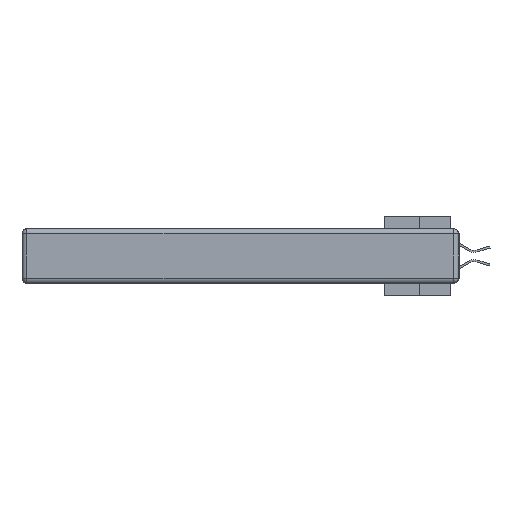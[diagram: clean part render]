
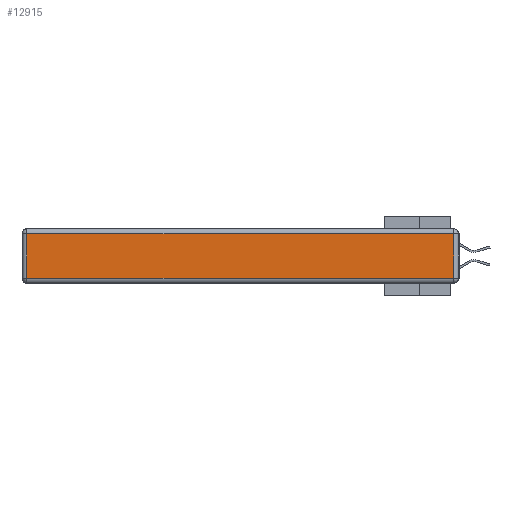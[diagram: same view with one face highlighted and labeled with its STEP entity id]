
A CAD part, left-side view. The second image highlights one B-rep face of the part: STEP entity #12915.
In plain terms, the highlighted planar face has unit normal (-1, 0, 0).
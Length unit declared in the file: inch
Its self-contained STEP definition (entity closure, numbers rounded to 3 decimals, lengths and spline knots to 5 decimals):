
#353 = EDGE_LOOP ( 'NONE', ( #5043, #460, #6641, #28069 ) ) ;
#437 = DIRECTION ( 'NONE',  ( -1., 0., 0. ) ) ;
#460 = ORIENTED_EDGE ( 'NONE', *, *, #6796, .T. ) ;
#1676 = FACE_OUTER_BOUND ( 'NONE', #353, .T. ) ;
#2303 = LINE ( 'NONE', #7377, #29376 ) ;
#2669 = PLANE ( 'NONE',  #26772 ) ;
#3069 = CARTESIAN_POINT ( 'NONE',  ( 0., 0., -0.343 ) ) ;
#3465 = VERTEX_POINT ( 'NONE', #5229 ) ;
#3587 = VECTOR ( 'NONE', #23182, 39.37008 ) ;
#4203 = CARTESIAN_POINT ( 'NONE',  ( 0., 0., -0.313 ) ) ;
#4297 = DIRECTION ( 'NONE',  ( 0., -1., 0. ) ) ;
#4678 = DIRECTION ( 'NONE',  ( 0., 1., 0. ) ) ;
#5043 = ORIENTED_EDGE ( 'NONE', *, *, #13978, .T. ) ;
#5229 = CARTESIAN_POINT ( 'NONE',  ( 0., 0.03, -0.313 ) ) ;
#5872 = VERTEX_POINT ( 'NONE', #11724 ) ;
#6641 = ORIENTED_EDGE ( 'NONE', *, *, #22964, .T. ) ;
#6796 = EDGE_CURVE ( 'NONE', #3465, #5872, #2303, .T. ) ;
#7377 = CARTESIAN_POINT ( 'NONE',  ( 0., 0.03, -0.343 ) ) ;
#8355 = LINE ( 'NONE', #11150, #3587 ) ;
#10765 = VERTEX_POINT ( 'NONE', #26553 ) ;
#11150 = CARTESIAN_POINT ( 'NONE',  ( 0., 2.72, -0.343 ) ) ;
#11654 = CARTESIAN_POINT ( 'NONE',  ( 0., 2.75, -0.03 ) ) ;
#11724 = CARTESIAN_POINT ( 'NONE',  ( 0., 0.03, -0.03 ) ) ;
#12848 = CARTESIAN_POINT ( 'NONE',  ( 0., 2.72, -0.313 ) ) ;
#12915 = ADVANCED_FACE ( 'NONE', ( #1676 ), #2669, .T. ) ;
#13978 = EDGE_CURVE ( 'NONE', #27571, #3465, #28650, .T. ) ;
#14248 = DIRECTION ( 'NONE',  ( 0., 0., 1. ) ) ;
#14354 = VECTOR ( 'NONE', #4678, 39.37008 ) ;
#22964 = EDGE_CURVE ( 'NONE', #5872, #10765, #24536, .T. ) ;
#23182 = DIRECTION ( 'NONE',  ( 0., 0., -1. ) ) ;
#24536 = LINE ( 'NONE', #11654, #14354 ) ;
#26553 = CARTESIAN_POINT ( 'NONE',  ( 0., 2.72, -0.03 ) ) ;
#26772 = AXIS2_PLACEMENT_3D ( 'NONE', #3069, #437, #28704 ) ;
#27571 = VERTEX_POINT ( 'NONE', #12848 ) ;
#27928 = VECTOR ( 'NONE', #4297, 39.37008 ) ;
#28069 = ORIENTED_EDGE ( 'NONE', *, *, #28497, .T. ) ;
#28497 = EDGE_CURVE ( 'NONE', #10765, #27571, #8355, .T. ) ;
#28650 = LINE ( 'NONE', #4203, #27928 ) ;
#28704 = DIRECTION ( 'NONE',  ( 0., 0., 1. ) ) ;
#29376 = VECTOR ( 'NONE', #14248, 39.37008 ) ;
